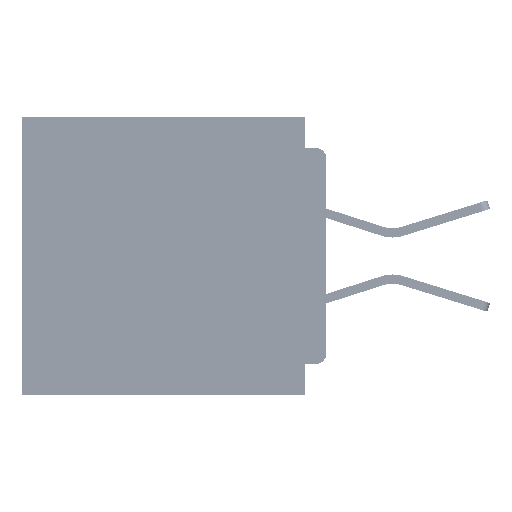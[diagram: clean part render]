
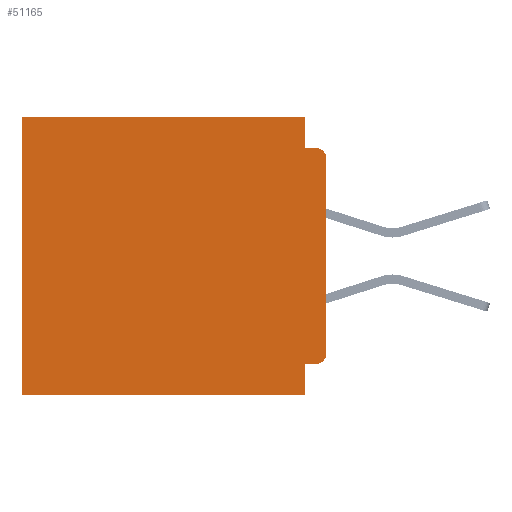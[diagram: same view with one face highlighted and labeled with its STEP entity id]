
A CAD part, left-side view. The second image highlights one B-rep face of the part: STEP entity #51165.
In plain terms, the highlighted planar face has unit normal (-1, 0, 0).
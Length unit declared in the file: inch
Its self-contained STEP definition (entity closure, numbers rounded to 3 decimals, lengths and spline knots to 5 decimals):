
#496 = ORIENTED_EDGE ( 'NONE', *, *, #20196, .F. ) ;
#824 = CARTESIAN_POINT ( 'NONE',  ( 0.3, 0.015, -0.34 ) ) ;
#1395 = CARTESIAN_POINT ( 'NONE',  ( 0.3, 0.015, -0.045 ) ) ;
#1490 = DIRECTION ( 'NONE',  ( 0., -1., 0. ) ) ;
#2655 = VERTEX_POINT ( 'NONE', #62435 ) ;
#3373 = VERTEX_POINT ( 'NONE', #40348 ) ;
#4270 = ORIENTED_EDGE ( 'NONE', *, *, #46197, .F. ) ;
#4859 = EDGE_CURVE ( 'NONE', #36604, #3373, #13160, .T. ) ;
#5099 = LINE ( 'NONE', #54627, #46636 ) ;
#5387 = DIRECTION ( 'NONE',  ( 1., 0., 0. ) ) ;
#5840 = LINE ( 'NONE', #34030, #64935 ) ;
#6337 = DIRECTION ( 'NONE',  ( 0., 0., -1. ) ) ;
#6712 = CARTESIAN_POINT ( 'NONE',  ( 0.3, 0.015, -0.06 ) ) ;
#8210 = ORIENTED_EDGE ( 'NONE', *, *, #12415, .F. ) ;
#10492 = VERTEX_POINT ( 'NONE', #31324 ) ;
#10541 = LINE ( 'NONE', #10812, #37701 ) ;
#10691 = VERTEX_POINT ( 'NONE', #49248 ) ;
#10812 = CARTESIAN_POINT ( 'NONE',  ( 0.3, 0.031, -0.4 ) ) ;
#11193 = VECTOR ( 'NONE', #64978, 39.37008 ) ;
#12032 = AXIS2_PLACEMENT_3D ( 'NONE', #6712, #44623, #12139 ) ;
#12139 = DIRECTION ( 'NONE',  ( 0., 0., -1. ) ) ;
#12415 = EDGE_CURVE ( 'NONE', #2655, #32215, #30688, .T. ) ;
#13160 = LINE ( 'NONE', #23911, #57967 ) ;
#13338 = ORIENTED_EDGE ( 'NONE', *, *, #23402, .T. ) ;
#14441 = CARTESIAN_POINT ( 'NONE',  ( 0.3, 0., -0.4 ) ) ;
#16226 = DIRECTION ( 'NONE',  ( 0., 0., -1. ) ) ;
#20196 = EDGE_CURVE ( 'NONE', #36604, #20620, #5099, .T. ) ;
#20620 = VERTEX_POINT ( 'NONE', #26210 ) ;
#20642 = CARTESIAN_POINT ( 'NONE',  ( 0.3, 0.437, -0.4 ) ) ;
#21119 = ORIENTED_EDGE ( 'NONE', *, *, #4859, .T. ) ;
#21875 = CARTESIAN_POINT ( 'NONE',  ( 0.3, 0., -0.4 ) ) ;
#22008 = ORIENTED_EDGE ( 'NONE', *, *, #63239, .T. ) ;
#22207 = LINE ( 'NONE', #21875, #11193 ) ;
#22472 = VECTOR ( 'NONE', #25859, 39.37008 ) ;
#23402 = EDGE_CURVE ( 'NONE', #3373, #32215, #36937, .T. ) ;
#23911 = CARTESIAN_POINT ( 'NONE',  ( 0.3, 0., 0. ) ) ;
#24059 = ORIENTED_EDGE ( 'NONE', *, *, #41945, .T. ) ;
#24831 = AXIS2_PLACEMENT_3D ( 'NONE', #824, #38840, #6337 ) ;
#25859 = DIRECTION ( 'NONE',  ( 0., 0., -1. ) ) ;
#26210 = CARTESIAN_POINT ( 'NONE',  ( 0.3, 0.031, -0.045 ) ) ;
#28879 = VERTEX_POINT ( 'NONE', #69452 ) ;
#29167 = CARTESIAN_POINT ( 'NONE',  ( 0.3, 0.437, -0.4 ) ) ;
#30280 = EDGE_CURVE ( 'NONE', #10492, #52305, #22207, .T. ) ;
#30688 = LINE ( 'NONE', #14441, #43397 ) ;
#31324 = CARTESIAN_POINT ( 'NONE',  ( 0.3, 0., -0.06 ) ) ;
#32215 = VERTEX_POINT ( 'NONE', #29167 ) ;
#32435 = PLANE ( 'NONE',  #61611 ) ;
#33161 = DIRECTION ( 'NONE',  ( 0., 0., -1. ) ) ;
#34030 = CARTESIAN_POINT ( 'NONE',  ( 0.3, 0., -0.045 ) ) ;
#35178 = EDGE_LOOP ( 'NONE', ( #63540, #22008, #57955, #496, #21119, #13338, #8210, #35266, #4270, #24059 ) ) ;
#35266 = ORIENTED_EDGE ( 'NONE', *, *, #54393, .F. ) ;
#35499 = CIRCLE ( 'NONE', #24831, 0.015 ) ;
#36316 = DIRECTION ( 'NONE',  ( 0., 1., 0. ) ) ;
#36604 = VERTEX_POINT ( 'NONE', #52764 ) ;
#36937 = LINE ( 'NONE', #20642, #22472 ) ;
#37701 = VECTOR ( 'NONE', #16226, 39.37008 ) ;
#38840 = DIRECTION ( 'NONE',  ( -1., 0., 0. ) ) ;
#39171 = VECTOR ( 'NONE', #69269, 39.37008 ) ;
#40348 = CARTESIAN_POINT ( 'NONE',  ( 0.3, 0.437, 0. ) ) ;
#41945 = EDGE_CURVE ( 'NONE', #10691, #52305, #35499, .T. ) ;
#43355 = DIRECTION ( 'NONE',  ( 0., 0., -1. ) ) ;
#43397 = VECTOR ( 'NONE', #36316, 39.37008 ) ;
#44623 = DIRECTION ( 'NONE',  ( -1., 0., 0. ) ) ;
#46197 = EDGE_CURVE ( 'NONE', #10691, #28879, #65992, .T. ) ;
#46486 = VERTEX_POINT ( 'NONE', #1395 ) ;
#46636 = VECTOR ( 'NONE', #33161, 39.37008 ) ;
#49248 = CARTESIAN_POINT ( 'NONE',  ( 0.3, 0.015, -0.355 ) ) ;
#51165 = ADVANCED_FACE ( 'NONE', ( #66723 ), #32435, .F. ) ;
#52305 = VERTEX_POINT ( 'NONE', #58183 ) ;
#52764 = CARTESIAN_POINT ( 'NONE',  ( 0.3, 0.031, 0. ) ) ;
#54393 = EDGE_CURVE ( 'NONE', #28879, #2655, #10541, .T. ) ;
#54627 = CARTESIAN_POINT ( 'NONE',  ( 0.3, 0.031, 0. ) ) ;
#56284 = DIRECTION ( 'NONE',  ( 0., 1., 0. ) ) ;
#57955 = ORIENTED_EDGE ( 'NONE', *, *, #66113, .F. ) ;
#57967 = VECTOR ( 'NONE', #56284, 39.37008 ) ;
#58183 = CARTESIAN_POINT ( 'NONE',  ( 0.3, 0., -0.34 ) ) ;
#58453 = CARTESIAN_POINT ( 'NONE',  ( 0.3, 0., -0.355 ) ) ;
#59808 = CIRCLE ( 'NONE', #12032, 0.015 ) ;
#61611 = AXIS2_PLACEMENT_3D ( 'NONE', #68362, #5387, #43355 ) ;
#62435 = CARTESIAN_POINT ( 'NONE',  ( 0.3, 0.031, -0.4 ) ) ;
#63239 = EDGE_CURVE ( 'NONE', #10492, #46486, #59808, .T. ) ;
#63540 = ORIENTED_EDGE ( 'NONE', *, *, #30280, .F. ) ;
#64935 = VECTOR ( 'NONE', #1490, 39.37008 ) ;
#64978 = DIRECTION ( 'NONE',  ( 0., 0., -1. ) ) ;
#65992 = LINE ( 'NONE', #58453, #39171 ) ;
#66113 = EDGE_CURVE ( 'NONE', #20620, #46486, #5840, .T. ) ;
#66723 = FACE_OUTER_BOUND ( 'NONE', #35178, .T. ) ;
#68362 = CARTESIAN_POINT ( 'NONE',  ( 0.3, 0., -0.4 ) ) ;
#69269 = DIRECTION ( 'NONE',  ( 0., 1., 0. ) ) ;
#69452 = CARTESIAN_POINT ( 'NONE',  ( 0.3, 0.031, -0.355 ) ) ;
